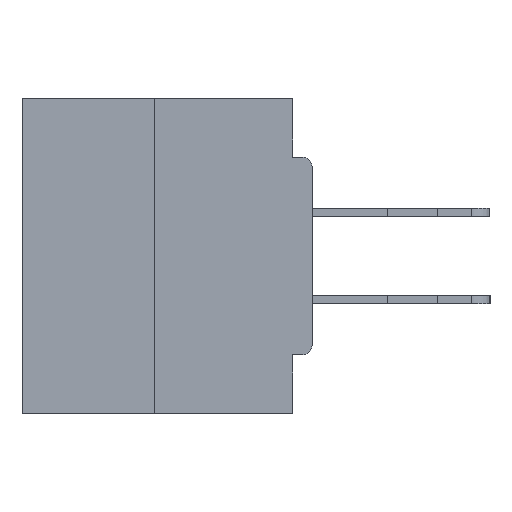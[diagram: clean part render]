
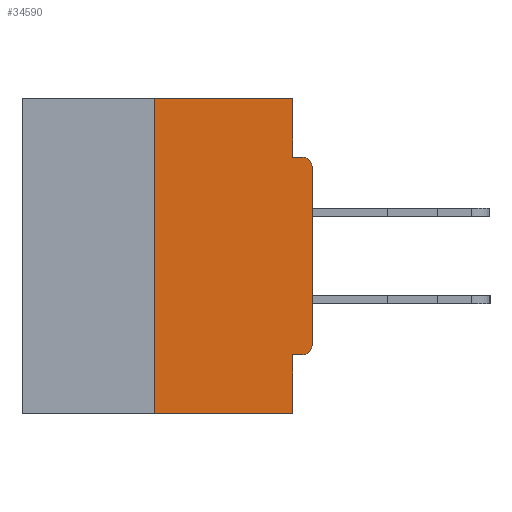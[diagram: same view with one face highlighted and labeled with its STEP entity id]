
A CAD part, left-side view. The second image highlights one B-rep face of the part: STEP entity #34590.
In plain terms, the highlighted planar face has unit normal (-1, 0, 0).
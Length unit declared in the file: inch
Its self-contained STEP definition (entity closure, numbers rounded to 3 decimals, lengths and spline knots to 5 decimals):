
#13 = DIRECTION ( 'NONE',  ( 1., 0., 0. ) ) ;
#111 = LINE ( 'NONE', #20149, #27115 ) ;
#428 = CARTESIAN_POINT ( 'NONE',  ( 0., 0.031, -0.4065 ) ) ;
#1540 = EDGE_CURVE ( 'NONE', #25648, #26091, #23533, .T. ) ;
#1908 = LINE ( 'NONE', #24519, #11470 ) ;
#2307 = VERTEX_POINT ( 'NONE', #5023 ) ;
#2713 = CARTESIAN_POINT ( 'NONE',  ( 0., 0.031, -0.0935 ) ) ;
#3151 = CARTESIAN_POINT ( 'NONE',  ( 0., 0., -0.1085 ) ) ;
#3385 = ORIENTED_EDGE ( 'NONE', *, *, #1540, .F. ) ;
#3978 = ORIENTED_EDGE ( 'NONE', *, *, #4505, .F. ) ;
#4047 = EDGE_CURVE ( 'NONE', #2307, #33733, #10662, .T. ) ;
#4429 = DIRECTION ( 'NONE',  ( 0., 0., -1. ) ) ;
#4505 = EDGE_CURVE ( 'NONE', #26091, #12849, #111, .T. ) ;
#4648 = LINE ( 'NONE', #18970, #9530 ) ;
#4926 = VERTEX_POINT ( 'NONE', #3151 ) ;
#5023 = CARTESIAN_POINT ( 'NONE',  ( 0., 0.015, -0.4065 ) ) ;
#5051 = ORIENTED_EDGE ( 'NONE', *, *, #4047, .T. ) ;
#5259 = DIRECTION ( 'NONE',  ( -1., 0., 0. ) ) ;
#5555 = CARTESIAN_POINT ( 'NONE',  ( 0., 0.46, 0. ) ) ;
#6082 = PLANE ( 'NONE',  #13233 ) ;
#6167 = ORIENTED_EDGE ( 'NONE', *, *, #13273, .T. ) ;
#7433 = VECTOR ( 'NONE', #4429, 39.37008 ) ;
#7574 = ORIENTED_EDGE ( 'NONE', *, *, #26920, .T. ) ;
#8411 = CARTESIAN_POINT ( 'NONE',  ( 0., 0., -0.4065 ) ) ;
#8905 = ORIENTED_EDGE ( 'NONE', *, *, #18138, .T. ) ;
#9530 = VECTOR ( 'NONE', #29446, 39.37008 ) ;
#9940 = EDGE_CURVE ( 'NONE', #17466, #25648, #4648, .T. ) ;
#10060 = CARTESIAN_POINT ( 'NONE',  ( 0., 0.46, -0.5 ) ) ;
#10662 = CIRCLE ( 'NONE', #26477, 0.015 ) ;
#10827 = ORIENTED_EDGE ( 'NONE', *, *, #9940, .F. ) ;
#10978 = CARTESIAN_POINT ( 'NONE',  ( 0., 0.25, 0. ) ) ;
#11457 = VECTOR ( 'NONE', #33550, 39.37008 ) ;
#11470 = VECTOR ( 'NONE', #21404, 39.37008 ) ;
#11591 = CARTESIAN_POINT ( 'NONE',  ( 0., 0.015, -0.1085 ) ) ;
#11863 = CARTESIAN_POINT ( 'NONE',  ( 0., 0.015, -0.0935 ) ) ;
#12486 = DIRECTION ( 'NONE',  ( 0., 0., -1. ) ) ;
#12849 = VERTEX_POINT ( 'NONE', #11863 ) ;
#13233 = AXIS2_PLACEMENT_3D ( 'NONE', #5555, #13, #28147 ) ;
#13273 = EDGE_CURVE ( 'NONE', #4926, #12849, #15836, .T. ) ;
#13669 = CARTESIAN_POINT ( 'NONE',  ( 0., 0.25, -0.5 ) ) ;
#14474 = VECTOR ( 'NONE', #14932, 39.37008 ) ;
#14932 = DIRECTION ( 'NONE',  ( 0., 0., 1. ) ) ;
#15836 = CIRCLE ( 'NONE', #28163, 0.015 ) ;
#17184 = EDGE_CURVE ( 'NONE', #31611, #17466, #25088, .T. ) ;
#17466 = VERTEX_POINT ( 'NONE', #35542 ) ;
#18132 = LINE ( 'NONE', #10060, #26744 ) ;
#18138 = EDGE_CURVE ( 'NONE', #31611, #31941, #18132, .T. ) ;
#18970 = CARTESIAN_POINT ( 'NONE',  ( 0., 0.46, 0. ) ) ;
#19167 = FACE_OUTER_BOUND ( 'NONE', #32382, .T. ) ;
#20149 = CARTESIAN_POINT ( 'NONE',  ( 0., 0., -0.0935 ) ) ;
#20344 = EDGE_CURVE ( 'NONE', #2307, #34161, #33580, .T. ) ;
#21404 = DIRECTION ( 'NONE',  ( 0., 0., -1. ) ) ;
#21853 = CARTESIAN_POINT ( 'NONE',  ( 0., 0., -0.3915 ) ) ;
#22785 = DIRECTION ( 'NONE',  ( -1., 0., 0. ) ) ;
#23533 = LINE ( 'NONE', #23717, #7433 ) ;
#23717 = CARTESIAN_POINT ( 'NONE',  ( 0., 0.031, 0. ) ) ;
#24519 = CARTESIAN_POINT ( 'NONE',  ( 0., 0.031, -0.5 ) ) ;
#24767 = CARTESIAN_POINT ( 'NONE',  ( 0., 0.031, -0.5 ) ) ;
#25088 = LINE ( 'NONE', #10978, #11457 ) ;
#25474 = DIRECTION ( 'NONE',  ( 0., -1., 0. ) ) ;
#25648 = VERTEX_POINT ( 'NONE', #31394 ) ;
#26091 = VERTEX_POINT ( 'NONE', #2713 ) ;
#26477 = AXIS2_PLACEMENT_3D ( 'NONE', #32294, #5259, #12486 ) ;
#26744 = VECTOR ( 'NONE', #28985, 39.37008 ) ;
#26920 = EDGE_CURVE ( 'NONE', #33733, #4926, #28885, .T. ) ;
#27115 = VECTOR ( 'NONE', #25474, 39.37008 ) ;
#27475 = ORIENTED_EDGE ( 'NONE', *, *, #34088, .F. ) ;
#27894 = DIRECTION ( 'NONE',  ( 0., 1., 0. ) ) ;
#28147 = DIRECTION ( 'NONE',  ( 0., 0., -1. ) ) ;
#28163 = AXIS2_PLACEMENT_3D ( 'NONE', #11591, #22785, #33993 ) ;
#28885 = LINE ( 'NONE', #34767, #14474 ) ;
#28985 = DIRECTION ( 'NONE',  ( 0., -1., 0. ) ) ;
#29249 = ORIENTED_EDGE ( 'NONE', *, *, #20344, .F. ) ;
#29446 = DIRECTION ( 'NONE',  ( 0., -1., 0. ) ) ;
#30937 = VECTOR ( 'NONE', #27894, 39.37008 ) ;
#31394 = CARTESIAN_POINT ( 'NONE',  ( 0., 0.031, 0. ) ) ;
#31611 = VERTEX_POINT ( 'NONE', #13669 ) ;
#31941 = VERTEX_POINT ( 'NONE', #24767 ) ;
#32294 = CARTESIAN_POINT ( 'NONE',  ( 0., 0.015, -0.3915 ) ) ;
#32382 = EDGE_LOOP ( 'NONE', ( #10827, #35484, #8905, #27475, #29249, #5051, #7574, #6167, #3978, #3385 ) ) ;
#33550 = DIRECTION ( 'NONE',  ( 0., 0., 1. ) ) ;
#33580 = LINE ( 'NONE', #8411, #30937 ) ;
#33733 = VERTEX_POINT ( 'NONE', #21853 ) ;
#33993 = DIRECTION ( 'NONE',  ( 0., 0., -1. ) ) ;
#34088 = EDGE_CURVE ( 'NONE', #34161, #31941, #1908, .T. ) ;
#34161 = VERTEX_POINT ( 'NONE', #428 ) ;
#34590 = ADVANCED_FACE ( 'NONE', ( #19167 ), #6082, .F. ) ;
#34767 = CARTESIAN_POINT ( 'NONE',  ( 0., 0., 0. ) ) ;
#35484 = ORIENTED_EDGE ( 'NONE', *, *, #17184, .F. ) ;
#35542 = CARTESIAN_POINT ( 'NONE',  ( 0., 0.25, 0. ) ) ;
